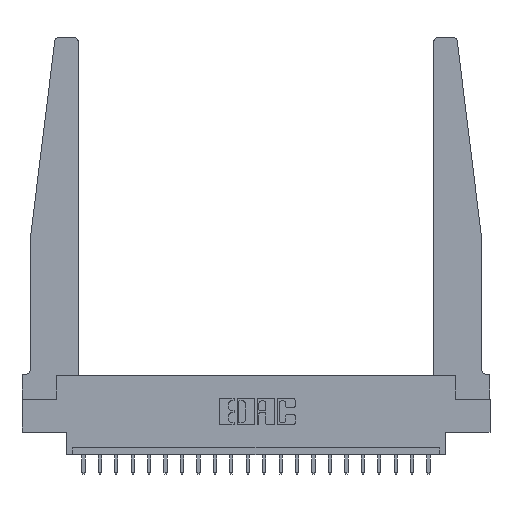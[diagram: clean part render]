
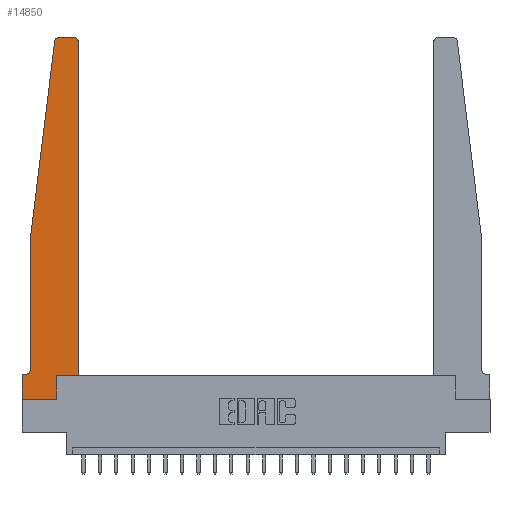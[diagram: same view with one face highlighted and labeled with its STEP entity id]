
A CAD part, top view. The second image highlights one B-rep face of the part: STEP entity #14850.
In plain terms, the highlighted planar face has unit normal (0, 0, 1).
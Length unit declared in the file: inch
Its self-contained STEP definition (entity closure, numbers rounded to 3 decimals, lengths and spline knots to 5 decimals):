
#55 = ORIENTED_EDGE ( 'NONE', *, *, #9236, .T. ) ;
#118 = CARTESIAN_POINT ( 'NONE',  ( 0.27653, 2.75, 0.37 ) ) ;
#709 = LINE ( 'NONE', #7622, #19930 ) ;
#731 = ORIENTED_EDGE ( 'NONE', *, *, #6487, .T. ) ;
#894 = DIRECTION ( 'NONE',  ( 0., 1., 0. ) ) ;
#900 = DIRECTION ( 'NONE',  ( 0., -1., 0. ) ) ;
#1047 = CARTESIAN_POINT ( 'NONE',  ( 0.065, 1.25, 0.37 ) ) ;
#1367 = VECTOR ( 'NONE', #15352, 39.37008 ) ;
#2012 = DIRECTION ( 'NONE',  ( 0., 0., 1. ) ) ;
#2185 = LINE ( 'NONE', #3601, #1367 ) ;
#2416 = CARTESIAN_POINT ( 'NONE',  ( 0., 0.1875, 0.37 ) ) ;
#2532 = LINE ( 'NONE', #19319, #12944 ) ;
#3001 = CARTESIAN_POINT ( 'NONE',  ( 0.425, 0.18, 0.37 ) ) ;
#3180 = DIRECTION ( 'NONE',  ( 0., 0., 1. ) ) ;
#3581 = ORIENTED_EDGE ( 'NONE', *, *, #9687, .T. ) ;
#3601 = CARTESIAN_POINT ( 'NONE',  ( 0.065, 0.1875, 0.37 ) ) ;
#3681 = AXIS2_PLACEMENT_3D ( 'NONE', #11679, #2012, #8280 ) ;
#4523 = EDGE_LOOP ( 'NONE', ( #731, #9931, #10810, #13858, #17803, #20733, #5903, #16371, #55, #19968, #3581, #15516 ) ) ;
#4621 = CARTESIAN_POINT ( 'NONE',  ( 0.395, 2.72, 0.37 ) ) ;
#4785 = LINE ( 'NONE', #21360, #5734 ) ;
#5734 = VECTOR ( 'NONE', #19593, 39.37008 ) ;
#5903 = ORIENTED_EDGE ( 'NONE', *, *, #16336, .T. ) ;
#6066 = CARTESIAN_POINT ( 'NONE',  ( 0.25, 2.75, 0.37 ) ) ;
#6152 = CIRCLE ( 'NONE', #3681, 0.03 ) ;
#6487 = EDGE_CURVE ( 'NONE', #8304, #19345, #11233, .T. ) ;
#6595 = CIRCLE ( 'NONE', #15685, 0.05 ) ;
#6781 = CARTESIAN_POINT ( 'NONE',  ( 0.2605, 0.18, 0.37 ) ) ;
#6894 = CARTESIAN_POINT ( 'NONE',  ( 0., 0., 0.37 ) ) ;
#6931 = VERTEX_POINT ( 'NONE', #2416 ) ;
#7078 = PLANE ( 'NONE',  #21499 ) ;
#7243 = EDGE_CURVE ( 'NONE', #13351, #6931, #2185, .T. ) ;
#7608 = DIRECTION ( 'NONE',  ( -1., 0., 0. ) ) ;
#7622 = CARTESIAN_POINT ( 'NONE',  ( 0.2605, 0.18, 0.37 ) ) ;
#7708 = CARTESIAN_POINT ( 'NONE',  ( 0., 0., 0.37 ) ) ;
#7717 = LINE ( 'NONE', #16159, #18027 ) ;
#7860 = DIRECTION ( 'NONE',  ( -0.122, -0.992, 0. ) ) ;
#8280 = DIRECTION ( 'NONE',  ( 1., 0., 0. ) ) ;
#8304 = VERTEX_POINT ( 'NONE', #17242 ) ;
#8745 = CARTESIAN_POINT ( 'NONE',  ( 0.065, 0.2375, 0.37 ) ) ;
#8994 = VERTEX_POINT ( 'NONE', #8745 ) ;
#9136 = CARTESIAN_POINT ( 'NONE',  ( 0.065, 1.25, 0.37 ) ) ;
#9236 = EDGE_CURVE ( 'NONE', #17525, #14088, #709, .T. ) ;
#9359 = DIRECTION ( 'NONE',  ( 0., -1., 0. ) ) ;
#9477 = LINE ( 'NONE', #7708, #12048 ) ;
#9687 = EDGE_CURVE ( 'NONE', #21123, #13933, #2532, .T. ) ;
#9694 = DIRECTION ( 'NONE',  ( 1., 0., 0. ) ) ;
#9789 = CARTESIAN_POINT ( 'NONE',  ( 0.015, 0.2375, 0.37 ) ) ;
#9842 = CIRCLE ( 'NONE', #21011, 0.03 ) ;
#9931 = ORIENTED_EDGE ( 'NONE', *, *, #19093, .T. ) ;
#9997 = DIRECTION ( 'NONE',  ( -1., 0., 0. ) ) ;
#10230 = CARTESIAN_POINT ( 'NONE',  ( 0., 0., 0.37 ) ) ;
#10488 = DIRECTION ( 'NONE',  ( 0., 0., 1. ) ) ;
#10588 = DIRECTION ( 'NONE',  ( 1., 0., 0. ) ) ;
#10649 = VECTOR ( 'NONE', #16762, 39.37008 ) ;
#10810 = ORIENTED_EDGE ( 'NONE', *, *, #21040, .T. ) ;
#10844 = EDGE_CURVE ( 'NONE', #13933, #8304, #9842, .T. ) ;
#10982 = VERTEX_POINT ( 'NONE', #10230 ) ;
#11233 = LINE ( 'NONE', #6066, #17096 ) ;
#11312 = DIRECTION ( 'NONE',  ( 0., 0., -1. ) ) ;
#11679 = CARTESIAN_POINT ( 'NONE',  ( 0.27653, 2.72, 0.37 ) ) ;
#12048 = VECTOR ( 'NONE', #9359, 39.37008 ) ;
#12121 = CARTESIAN_POINT ( 'NONE',  ( 0., 0.1875, 0.37 ) ) ;
#12944 = VECTOR ( 'NONE', #894, 39.37008 ) ;
#13351 = VERTEX_POINT ( 'NONE', #18358 ) ;
#13858 = ORIENTED_EDGE ( 'NONE', *, *, #18104, .T. ) ;
#13933 = VERTEX_POINT ( 'NONE', #18985 ) ;
#14088 = VERTEX_POINT ( 'NONE', #6781 ) ;
#14850 = ADVANCED_FACE ( 'NONE', ( #15415 ), #7078, .T. ) ;
#15226 = LINE ( 'NONE', #6894, #10649 ) ;
#15352 = DIRECTION ( 'NONE',  ( -1., 0., 0. ) ) ;
#15415 = FACE_OUTER_BOUND ( 'NONE', #4523, .T. ) ;
#15516 = ORIENTED_EDGE ( 'NONE', *, *, #10844, .T. ) ;
#15631 = DIRECTION ( 'NONE',  ( 0., 1., 0. ) ) ;
#15634 = CARTESIAN_POINT ( 'NONE',  ( 0.2605, 0., 0.37 ) ) ;
#15685 = AXIS2_PLACEMENT_3D ( 'NONE', #9789, #11312, #9997 ) ;
#16159 = CARTESIAN_POINT ( 'NONE',  ( 0.065, 1.25, 0.37 ) ) ;
#16336 = EDGE_CURVE ( 'NONE', #6931, #10982, #9477, .T. ) ;
#16371 = ORIENTED_EDGE ( 'NONE', *, *, #16975, .T. ) ;
#16715 = VECTOR ( 'NONE', #7860, 39.37008 ) ;
#16762 = DIRECTION ( 'NONE',  ( 1., 0., 0. ) ) ;
#16975 = EDGE_CURVE ( 'NONE', #10982, #17525, #15226, .T. ) ;
#17096 = VECTOR ( 'NONE', #7608, 39.37008 ) ;
#17170 = EDGE_CURVE ( 'NONE', #14088, #21123, #4785, .T. ) ;
#17242 = CARTESIAN_POINT ( 'NONE',  ( 0.395, 2.75, 0.37 ) ) ;
#17525 = VERTEX_POINT ( 'NONE', #15634 ) ;
#17803 = ORIENTED_EDGE ( 'NONE', *, *, #21512, .T. ) ;
#18027 = VECTOR ( 'NONE', #900, 39.37008 ) ;
#18104 = EDGE_CURVE ( 'NONE', #21294, #8994, #7717, .T. ) ;
#18358 = CARTESIAN_POINT ( 'NONE',  ( 0.015, 0.1875, 0.37 ) ) ;
#18592 = VERTEX_POINT ( 'NONE', #19597 ) ;
#18985 = CARTESIAN_POINT ( 'NONE',  ( 0.425, 2.72, 0.37 ) ) ;
#19093 = EDGE_CURVE ( 'NONE', #19345, #18592, #6152, .T. ) ;
#19319 = CARTESIAN_POINT ( 'NONE',  ( 0.425, 0.18, 0.37 ) ) ;
#19345 = VERTEX_POINT ( 'NONE', #118 ) ;
#19593 = DIRECTION ( 'NONE',  ( 1., 0., 0. ) ) ;
#19597 = CARTESIAN_POINT ( 'NONE',  ( 0.24675, 2.72367, 0.37 ) ) ;
#19930 = VECTOR ( 'NONE', #15631, 39.37008 ) ;
#19968 = ORIENTED_EDGE ( 'NONE', *, *, #17170, .T. ) ;
#20733 = ORIENTED_EDGE ( 'NONE', *, *, #7243, .T. ) ;
#21011 = AXIS2_PLACEMENT_3D ( 'NONE', #4621, #3180, #9694 ) ;
#21012 = LINE ( 'NONE', #1047, #16715 ) ;
#21040 = EDGE_CURVE ( 'NONE', #18592, #21294, #21012, .T. ) ;
#21123 = VERTEX_POINT ( 'NONE', #3001 ) ;
#21294 = VERTEX_POINT ( 'NONE', #9136 ) ;
#21360 = CARTESIAN_POINT ( 'NONE',  ( 0.425, 0.18, 0.37 ) ) ;
#21499 = AXIS2_PLACEMENT_3D ( 'NONE', #12121, #10488, #10588 ) ;
#21512 = EDGE_CURVE ( 'NONE', #8994, #13351, #6595, .T. ) ;
